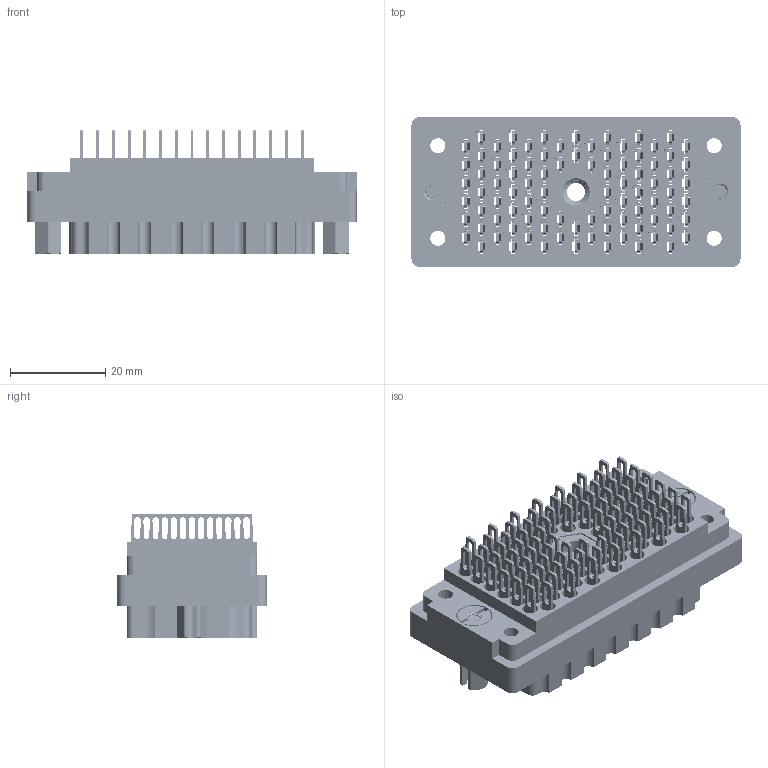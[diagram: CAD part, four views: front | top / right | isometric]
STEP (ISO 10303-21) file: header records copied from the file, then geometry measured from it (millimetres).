
FILE_DESCRIPTION (( 'STEP AP203' ), '1' );
FILE_NAME ('516-090-500-602.STEP', '2020-03-06T17:58:29', ( '' ), ( '' ), 'SwSTEP 2.0', 'SolidWorks 2016', '' );
FILE_SCHEMA (( 'CONFIG_CONTROL_DESIGN' ));
Length unit declared in the file: inch
Products named in the file (7): 516-221-090-102_090; 516-292-001_500 Contact; 516-252-091-102; 516 Part Receptacle_090; 516-252-095-100; 516-221-090-102_091; 516-090-500-602
Assembly tree (96 placements, depth 2):
  516-090-500-602
    516 Part Receptacle_090
    516-292-001_500 Contact  x90
    516-252-091-102  x2
    516-221-090-102_090
    516-252-095-100
    516-221-090-102_091
Bounding box: 69.04 x 31.34 x 26.21 mm (x, y, z)
Volume: 23887 mm3; surface area: 47406.7 mm2
Topology: 96 solids, 96 shells, 8971 faces, 26067 edges, 17305 vertices
Faces by surface type: plane 5302, cylinder 3055, bspline 568, cone 46
Entity records: 83758 total; most frequent: CARTESIAN_POINT 20809, ORIENTED_EDGE 12810, DIRECTION 12298, EDGE_CURVE 6405, LINE 4546, VECTOR 4546, VERTEX_POINT 4259, AXIS2_PLACEMENT_3D 3876
